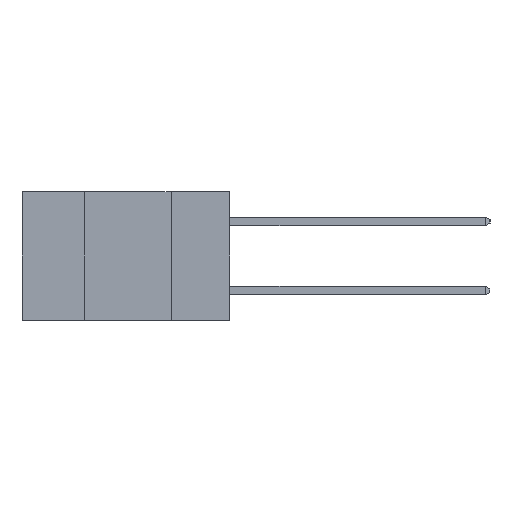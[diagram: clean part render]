
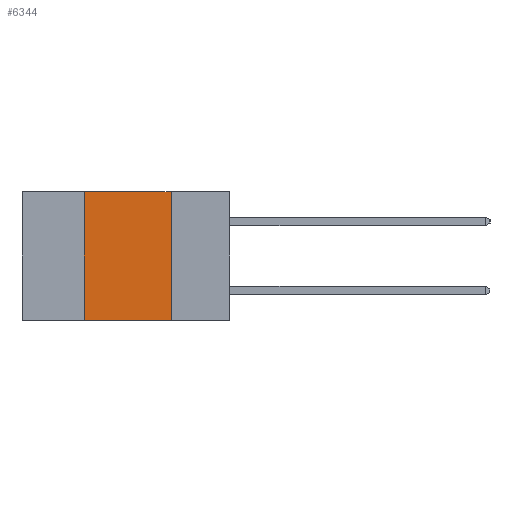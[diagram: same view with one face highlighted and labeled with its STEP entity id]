
A CAD part, left-side view. The second image highlights one B-rep face of the part: STEP entity #6344.
In plain terms, the highlighted planar face has unit normal (-1, 0, 0).
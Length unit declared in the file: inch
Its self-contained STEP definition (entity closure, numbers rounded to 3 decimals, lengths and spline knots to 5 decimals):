
#325 = VECTOR ( 'NONE', #9172, 39.37008 ) ;
#564 = DIRECTION ( 'NONE',  ( 0., -1., 0. ) ) ;
#614 = EDGE_CURVE ( 'NONE', #8398, #7826, #10310, .T. ) ;
#693 = FACE_OUTER_BOUND ( 'NONE', #5721, .T. ) ;
#938 = CARTESIAN_POINT ( 'NONE',  ( 0., 0.42, 0. ) ) ;
#1262 = VECTOR ( 'NONE', #9564, 39.37008 ) ;
#1781 = ORIENTED_EDGE ( 'NONE', *, *, #1993, .F. ) ;
#1897 = CARTESIAN_POINT ( 'NONE',  ( 0., 0.42, -0.37 ) ) ;
#1993 = EDGE_CURVE ( 'NONE', #6383, #7826, #4901, .T. ) ;
#3492 = VECTOR ( 'NONE', #564, 39.37008 ) ;
#4441 = EDGE_CURVE ( 'NONE', #7712, #6383, #8515, .T. ) ;
#4901 = LINE ( 'NONE', #6676, #9449 ) ;
#4980 = ORIENTED_EDGE ( 'NONE', *, *, #4441, .F. ) ;
#5721 = EDGE_LOOP ( 'NONE', ( #1781, #4980, #6915, #9656 ) ) ;
#6056 = CARTESIAN_POINT ( 'NONE',  ( 0., 0.6, 0. ) ) ;
#6098 = DIRECTION ( 'NONE',  ( 0., 0., -1. ) ) ;
#6143 = EDGE_CURVE ( 'NONE', #8398, #7712, #7585, .T. ) ;
#6344 = ADVANCED_FACE ( 'NONE', ( #693 ), #9443, .F. ) ;
#6383 = VERTEX_POINT ( 'NONE', #7868 ) ;
#6676 = CARTESIAN_POINT ( 'NONE',  ( 0., 0.17, 0. ) ) ;
#6915 = ORIENTED_EDGE ( 'NONE', *, *, #6143, .F. ) ;
#7585 = LINE ( 'NONE', #9205, #325 ) ;
#7712 = VERTEX_POINT ( 'NONE', #938 ) ;
#7826 = VERTEX_POINT ( 'NONE', #9739 ) ;
#7868 = CARTESIAN_POINT ( 'NONE',  ( 0., 0.17, 0. ) ) ;
#8398 = VERTEX_POINT ( 'NONE', #1897 ) ;
#8515 = LINE ( 'NONE', #9576, #1262 ) ;
#9126 = CARTESIAN_POINT ( 'NONE',  ( 0., 0.6, -0.37 ) ) ;
#9172 = DIRECTION ( 'NONE',  ( 0., 0., 1. ) ) ;
#9205 = CARTESIAN_POINT ( 'NONE',  ( 0., 0.42, 0. ) ) ;
#9321 = AXIS2_PLACEMENT_3D ( 'NONE', #6056, #11098, #6098 ) ;
#9443 = PLANE ( 'NONE',  #9321 ) ;
#9449 = VECTOR ( 'NONE', #11071, 39.37008 ) ;
#9564 = DIRECTION ( 'NONE',  ( 0., -1., 0. ) ) ;
#9576 = CARTESIAN_POINT ( 'NONE',  ( 0., 0.6, 0. ) ) ;
#9656 = ORIENTED_EDGE ( 'NONE', *, *, #614, .T. ) ;
#9739 = CARTESIAN_POINT ( 'NONE',  ( 0., 0.17, -0.37 ) ) ;
#10310 = LINE ( 'NONE', #9126, #3492 ) ;
#11071 = DIRECTION ( 'NONE',  ( 0., 0., -1. ) ) ;
#11098 = DIRECTION ( 'NONE',  ( 1., 0., 0. ) ) ;
